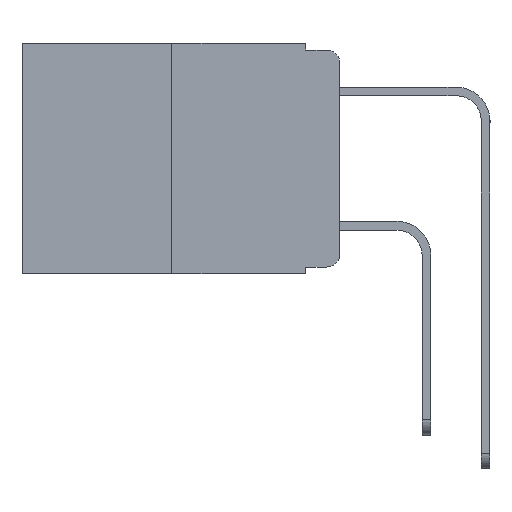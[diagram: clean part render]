
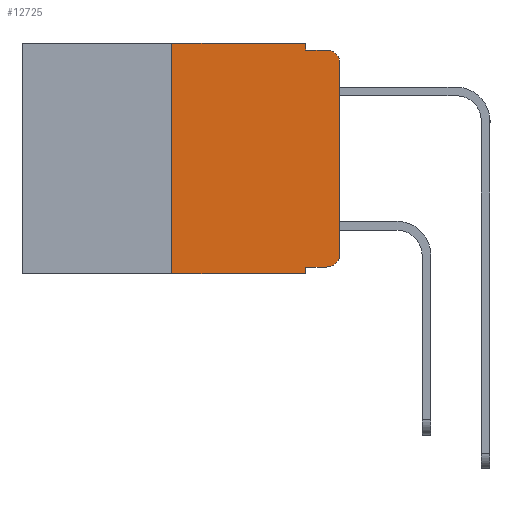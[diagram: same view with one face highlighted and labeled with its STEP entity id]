
A CAD part, left-side view. The second image highlights one B-rep face of the part: STEP entity #12725.
In plain terms, the highlighted planar face has unit normal (-1, 0, 0).
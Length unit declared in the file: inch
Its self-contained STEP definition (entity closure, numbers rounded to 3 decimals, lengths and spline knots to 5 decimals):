
#47 = AXIS2_PLACEMENT_3D ( 'NONE', #9188, #15784, #5917 ) ;
#230 = CARTESIAN_POINT ( 'NONE',  ( 0., 0.02, -0.333 ) ) ;
#916 = CARTESIAN_POINT ( 'NONE',  ( 0., 0., -0.313 ) ) ;
#935 = PLANE ( 'NONE',  #47 ) ;
#1054 = ORIENTED_EDGE ( 'NONE', *, *, #8378, .F. ) ;
#1285 = CARTESIAN_POINT ( 'NONE',  ( 0., 0.051, 0. ) ) ;
#1708 = LINE ( 'NONE', #17484, #18104 ) ;
#2089 = VECTOR ( 'NONE', #20861, 39.37008 ) ;
#2676 = CARTESIAN_POINT ( 'NONE',  ( 0., 0., -0.03 ) ) ;
#2850 = VECTOR ( 'NONE', #2961, 39.37008 ) ;
#2961 = DIRECTION ( 'NONE',  ( 0., 0., -1. ) ) ;
#3205 = CARTESIAN_POINT ( 'NONE',  ( 0., 0., 0. ) ) ;
#3765 = CARTESIAN_POINT ( 'NONE',  ( 0., 0.02, -0.01 ) ) ;
#4142 = EDGE_LOOP ( 'NONE', ( #17096, #7760, #5011, #8642, #9940, #9248, #6375, #1054, #5956, #4280 ) ) ;
#4280 = ORIENTED_EDGE ( 'NONE', *, *, #5023, .T. ) ;
#4487 = DIRECTION ( 'NONE',  ( 0., -1., 0. ) ) ;
#4866 = CARTESIAN_POINT ( 'NONE',  ( 0., 0.02, -0.03 ) ) ;
#4883 = FACE_OUTER_BOUND ( 'NONE', #4142, .T. ) ;
#5011 = ORIENTED_EDGE ( 'NONE', *, *, #13944, .F. ) ;
#5023 = EDGE_CURVE ( 'NONE', #7117, #6750, #6560, .T. ) ;
#5368 = CARTESIAN_POINT ( 'NONE',  ( 0., 0.25, 0. ) ) ;
#5531 = CARTESIAN_POINT ( 'NONE',  ( 0., 0.02, -0.313 ) ) ;
#5533 = DIRECTION ( 'NONE',  ( -1., 0., 0. ) ) ;
#5577 = VECTOR ( 'NONE', #6618, 39.37008 ) ;
#5917 = DIRECTION ( 'NONE',  ( 0., 0., -1. ) ) ;
#5956 = ORIENTED_EDGE ( 'NONE', *, *, #6174, .T. ) ;
#6174 = EDGE_CURVE ( 'NONE', #12329, #7117, #6541, .T. ) ;
#6318 = VECTOR ( 'NONE', #7056, 39.37008 ) ;
#6375 = ORIENTED_EDGE ( 'NONE', *, *, #9780, .T. ) ;
#6453 = CARTESIAN_POINT ( 'NONE',  ( 0., 0.25, -0.343 ) ) ;
#6539 = DIRECTION ( 'NONE',  ( 0., 0., -1. ) ) ;
#6541 = LINE ( 'NONE', #7453, #14810 ) ;
#6560 = CIRCLE ( 'NONE', #17343, 0.02 ) ;
#6618 = DIRECTION ( 'NONE',  ( 0., 0., -1. ) ) ;
#6750 = VERTEX_POINT ( 'NONE', #916 ) ;
#6821 = LINE ( 'NONE', #5368, #6318 ) ;
#7056 = DIRECTION ( 'NONE',  ( 0., 0., 1. ) ) ;
#7117 = VERTEX_POINT ( 'NONE', #230 ) ;
#7453 = CARTESIAN_POINT ( 'NONE',  ( 0., 0.051, -0.333 ) ) ;
#7643 = VERTEX_POINT ( 'NONE', #13125 ) ;
#7760 = ORIENTED_EDGE ( 'NONE', *, *, #14997, .T. ) ;
#8331 = CARTESIAN_POINT ( 'NONE',  ( 0., 0.051, -0.01 ) ) ;
#8361 = CARTESIAN_POINT ( 'NONE',  ( 0., 0.051, 0. ) ) ;
#8378 = EDGE_CURVE ( 'NONE', #12329, #20904, #14383, .T. ) ;
#8642 = ORIENTED_EDGE ( 'NONE', *, *, #12848, .F. ) ;
#8894 = VECTOR ( 'NONE', #14347, 39.37008 ) ;
#9032 = CARTESIAN_POINT ( 'NONE',  ( 0., 0.051, -0.343 ) ) ;
#9074 = VERTEX_POINT ( 'NONE', #2676 ) ;
#9116 = DIRECTION ( 'NONE',  ( 0., -1., 0. ) ) ;
#9188 = CARTESIAN_POINT ( 'NONE',  ( 0., 0.473, 0. ) ) ;
#9248 = ORIENTED_EDGE ( 'NONE', *, *, #9499, .F. ) ;
#9410 = LINE ( 'NONE', #12714, #8894 ) ;
#9499 = EDGE_CURVE ( 'NONE', #19913, #7643, #6821, .T. ) ;
#9565 = VERTEX_POINT ( 'NONE', #13798 ) ;
#9780 = EDGE_CURVE ( 'NONE', #19913, #20904, #9410, .T. ) ;
#9940 = ORIENTED_EDGE ( 'NONE', *, *, #20512, .F. ) ;
#10020 = VERTEX_POINT ( 'NONE', #8331 ) ;
#10096 = AXIS2_PLACEMENT_3D ( 'NONE', #4866, #16383, #6539 ) ;
#10717 = CIRCLE ( 'NONE', #10096, 0.02 ) ;
#10881 = LINE ( 'NONE', #14459, #2089 ) ;
#12329 = VERTEX_POINT ( 'NONE', #21070 ) ;
#12714 = CARTESIAN_POINT ( 'NONE',  ( 0., 0.473, -0.343 ) ) ;
#12725 = ADVANCED_FACE ( 'NONE', ( #4883 ), #935, .F. ) ;
#12848 = EDGE_CURVE ( 'NONE', #9565, #10020, #19703, .T. ) ;
#13125 = CARTESIAN_POINT ( 'NONE',  ( 0., 0.25, 0. ) ) ;
#13798 = CARTESIAN_POINT ( 'NONE',  ( 0., 0.051, 0. ) ) ;
#13944 = EDGE_CURVE ( 'NONE', #10020, #14301, #1708, .T. ) ;
#14301 = VERTEX_POINT ( 'NONE', #3765 ) ;
#14347 = DIRECTION ( 'NONE',  ( 0., -1., 0. ) ) ;
#14383 = LINE ( 'NONE', #8361, #5577 ) ;
#14459 = CARTESIAN_POINT ( 'NONE',  ( 0., 0.473, 0. ) ) ;
#14810 = VECTOR ( 'NONE', #9116, 39.37008 ) ;
#14997 = EDGE_CURVE ( 'NONE', #9074, #14301, #10717, .T. ) ;
#15159 = VECTOR ( 'NONE', #16350, 39.37008 ) ;
#15763 = DIRECTION ( 'NONE',  ( 0., 0., -1. ) ) ;
#15784 = DIRECTION ( 'NONE',  ( 1., 0., 0. ) ) ;
#16350 = DIRECTION ( 'NONE',  ( 0., 0., 1. ) ) ;
#16383 = DIRECTION ( 'NONE',  ( -1., 0., 0. ) ) ;
#17096 = ORIENTED_EDGE ( 'NONE', *, *, #18212, .T. ) ;
#17343 = AXIS2_PLACEMENT_3D ( 'NONE', #5531, #5533, #15763 ) ;
#17484 = CARTESIAN_POINT ( 'NONE',  ( 0., 0.051, -0.01 ) ) ;
#18104 = VECTOR ( 'NONE', #4487, 39.37008 ) ;
#18212 = EDGE_CURVE ( 'NONE', #6750, #9074, #19893, .T. ) ;
#19703 = LINE ( 'NONE', #1285, #2850 ) ;
#19893 = LINE ( 'NONE', #3205, #15159 ) ;
#19913 = VERTEX_POINT ( 'NONE', #6453 ) ;
#20512 = EDGE_CURVE ( 'NONE', #7643, #9565, #10881, .T. ) ;
#20861 = DIRECTION ( 'NONE',  ( 0., -1., 0. ) ) ;
#20904 = VERTEX_POINT ( 'NONE', #9032 ) ;
#21070 = CARTESIAN_POINT ( 'NONE',  ( 0., 0.051, -0.333 ) ) ;
